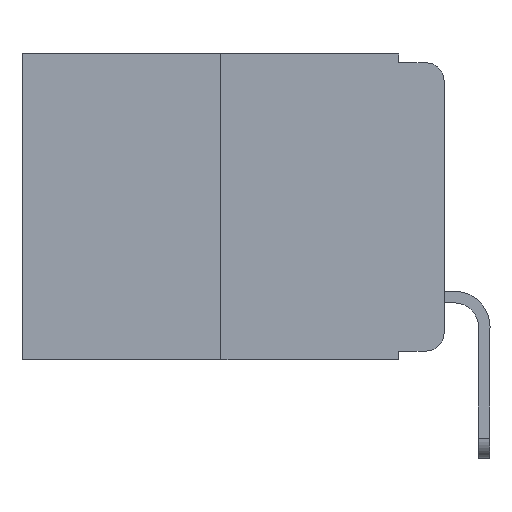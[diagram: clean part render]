
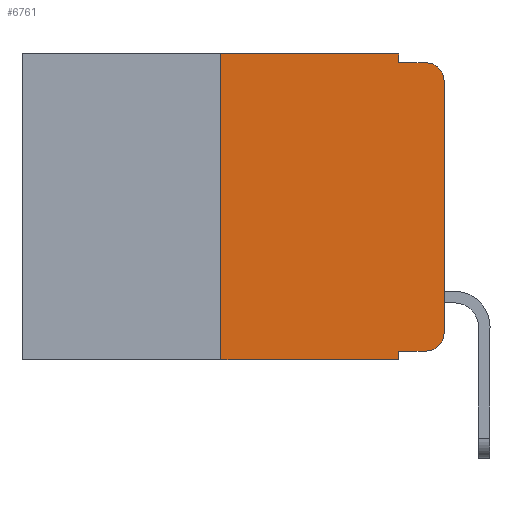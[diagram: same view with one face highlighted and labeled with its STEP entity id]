
A CAD part, left-side view. The second image highlights one B-rep face of the part: STEP entity #6761.
In plain terms, the highlighted planar face has unit normal (-1, 0, 0).
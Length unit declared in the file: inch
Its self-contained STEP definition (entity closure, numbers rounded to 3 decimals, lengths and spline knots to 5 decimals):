
#14 = CARTESIAN_POINT ( 'NONE',  ( 0., 0.25, -0.343 ) ) ;
#350 = VERTEX_POINT ( 'NONE', #11239 ) ;
#631 = EDGE_CURVE ( 'NONE', #5816, #4307, #10254, .T. ) ;
#965 = EDGE_CURVE ( 'NONE', #10689, #9677, #3555, .T. ) ;
#1026 = ORIENTED_EDGE ( 'NONE', *, *, #9726, .T. ) ;
#1250 = EDGE_CURVE ( 'NONE', #2884, #10689, #2243, .T. ) ;
#1435 = ORIENTED_EDGE ( 'NONE', *, *, #9919, .T. ) ;
#1567 = DIRECTION ( 'NONE',  ( -1., 0., 0. ) ) ;
#1580 = DIRECTION ( 'NONE',  ( 0., 0., 1. ) ) ;
#1717 = VECTOR ( 'NONE', #8645, 39.37008 ) ;
#1846 = VECTOR ( 'NONE', #8422, 39.37008 ) ;
#1937 = EDGE_CURVE ( 'NONE', #10510, #2884, #5516, .T. ) ;
#1985 = DIRECTION ( 'NONE',  ( 0., 0., -1. ) ) ;
#2203 = ORIENTED_EDGE ( 'NONE', *, *, #1250, .F. ) ;
#2243 = LINE ( 'NONE', #2761, #12134 ) ;
#2291 = EDGE_CURVE ( 'NONE', #4470, #10510, #10432, .T. ) ;
#2372 = DIRECTION ( 'NONE',  ( 0., -1., 0. ) ) ;
#2761 = CARTESIAN_POINT ( 'NONE',  ( 0., 0.051, 0. ) ) ;
#2884 = VERTEX_POINT ( 'NONE', #12487 ) ;
#2900 = AXIS2_PLACEMENT_3D ( 'NONE', #4416, #4414, #4397 ) ;
#2934 = ORIENTED_EDGE ( 'NONE', *, *, #2291, .F. ) ;
#2991 = AXIS2_PLACEMENT_3D ( 'NONE', #4071, #10620, #5057 ) ;
#3009 = CIRCLE ( 'NONE', #2900, 0.02 ) ;
#3310 = ORIENTED_EDGE ( 'NONE', *, *, #12541, .T. ) ;
#3372 = VERTEX_POINT ( 'NONE', #10532 ) ;
#3414 = CARTESIAN_POINT ( 'NONE',  ( 0., 0.25, 0. ) ) ;
#3555 = LINE ( 'NONE', #8073, #5907 ) ;
#3943 = DIRECTION ( 'NONE',  ( 0., -1., 0. ) ) ;
#4051 = CARTESIAN_POINT ( 'NONE',  ( 0., 0.051, -0.343 ) ) ;
#4071 = CARTESIAN_POINT ( 'NONE',  ( 0., 0.473, 0. ) ) ;
#4307 = VERTEX_POINT ( 'NONE', #4051 ) ;
#4397 = DIRECTION ( 'NONE',  ( 0., 0., -1. ) ) ;
#4414 = DIRECTION ( 'NONE',  ( -1., 0., 0. ) ) ;
#4416 = CARTESIAN_POINT ( 'NONE',  ( 0., 0.02, -0.313 ) ) ;
#4452 = CARTESIAN_POINT ( 'NONE',  ( 0., 0.051, 0. ) ) ;
#4470 = VERTEX_POINT ( 'NONE', #14 ) ;
#5057 = DIRECTION ( 'NONE',  ( 0., 0., -1. ) ) ;
#5123 = FACE_OUTER_BOUND ( 'NONE', #8836, .T. ) ;
#5149 = EDGE_CURVE ( 'NONE', #8551, #3372, #3009, .T. ) ;
#5220 = LINE ( 'NONE', #7090, #9912 ) ;
#5373 = CARTESIAN_POINT ( 'NONE',  ( 0., 0.051, -0.01 ) ) ;
#5375 = EDGE_CURVE ( 'NONE', #5816, #8551, #9433, .T. ) ;
#5516 = LINE ( 'NONE', #5775, #12467 ) ;
#5775 = CARTESIAN_POINT ( 'NONE',  ( 0., 0.473, 0. ) ) ;
#5816 = VERTEX_POINT ( 'NONE', #9638 ) ;
#5907 = VECTOR ( 'NONE', #2372, 39.37008 ) ;
#6761 = ADVANCED_FACE ( 'NONE', ( #5123 ), #9736, .F. ) ;
#7060 = ORIENTED_EDGE ( 'NONE', *, *, #965, .F. ) ;
#7090 = CARTESIAN_POINT ( 'NONE',  ( 0., 0.473, -0.343 ) ) ;
#7348 = LINE ( 'NONE', #7499, #1846 ) ;
#7499 = CARTESIAN_POINT ( 'NONE',  ( 0., 0., 0. ) ) ;
#7776 = CARTESIAN_POINT ( 'NONE',  ( 0., 0.02, -0.03 ) ) ;
#7948 = ORIENTED_EDGE ( 'NONE', *, *, #1937, .F. ) ;
#8038 = DIRECTION ( 'NONE',  ( 0., -1., 0. ) ) ;
#8039 = VECTOR ( 'NONE', #1580, 39.37008 ) ;
#8073 = CARTESIAN_POINT ( 'NONE',  ( 0., 0.051, -0.01 ) ) ;
#8074 = CIRCLE ( 'NONE', #8904, 0.02 ) ;
#8081 = CARTESIAN_POINT ( 'NONE',  ( 0., 0.02, -0.333 ) ) ;
#8139 = VECTOR ( 'NONE', #11029, 39.37008 ) ;
#8422 = DIRECTION ( 'NONE',  ( 0., 0., 1. ) ) ;
#8551 = VERTEX_POINT ( 'NONE', #8081 ) ;
#8645 = DIRECTION ( 'NONE',  ( 0., -1., 0. ) ) ;
#8687 = CARTESIAN_POINT ( 'NONE',  ( 0., 0.051, -0.333 ) ) ;
#8722 = DIRECTION ( 'NONE',  ( 0., 0., -1. ) ) ;
#8836 = EDGE_LOOP ( 'NONE', ( #1026, #1435, #7060, #2203, #7948, #2934, #3310, #11968, #12508, #11589 ) ) ;
#8904 = AXIS2_PLACEMENT_3D ( 'NONE', #7776, #1567, #8722 ) ;
#9433 = LINE ( 'NONE', #8687, #1717 ) ;
#9638 = CARTESIAN_POINT ( 'NONE',  ( 0., 0.051, -0.333 ) ) ;
#9677 = VERTEX_POINT ( 'NONE', #12756 ) ;
#9726 = EDGE_CURVE ( 'NONE', #3372, #350, #7348, .T. ) ;
#9736 = PLANE ( 'NONE',  #2991 ) ;
#9912 = VECTOR ( 'NONE', #8038, 39.37008 ) ;
#9919 = EDGE_CURVE ( 'NONE', #350, #9677, #8074, .T. ) ;
#10254 = LINE ( 'NONE', #4452, #8139 ) ;
#10432 = LINE ( 'NONE', #11322, #8039 ) ;
#10510 = VERTEX_POINT ( 'NONE', #3414 ) ;
#10532 = CARTESIAN_POINT ( 'NONE',  ( 0., 0., -0.313 ) ) ;
#10620 = DIRECTION ( 'NONE',  ( 1., 0., 0. ) ) ;
#10689 = VERTEX_POINT ( 'NONE', #5373 ) ;
#11029 = DIRECTION ( 'NONE',  ( 0., 0., -1. ) ) ;
#11239 = CARTESIAN_POINT ( 'NONE',  ( 0., 0., -0.03 ) ) ;
#11322 = CARTESIAN_POINT ( 'NONE',  ( 0., 0.25, 0. ) ) ;
#11589 = ORIENTED_EDGE ( 'NONE', *, *, #5149, .T. ) ;
#11968 = ORIENTED_EDGE ( 'NONE', *, *, #631, .F. ) ;
#12134 = VECTOR ( 'NONE', #1985, 39.37008 ) ;
#12467 = VECTOR ( 'NONE', #3943, 39.37008 ) ;
#12487 = CARTESIAN_POINT ( 'NONE',  ( 0., 0.051, 0. ) ) ;
#12508 = ORIENTED_EDGE ( 'NONE', *, *, #5375, .T. ) ;
#12541 = EDGE_CURVE ( 'NONE', #4470, #4307, #5220, .T. ) ;
#12756 = CARTESIAN_POINT ( 'NONE',  ( 0., 0.02, -0.01 ) ) ;
